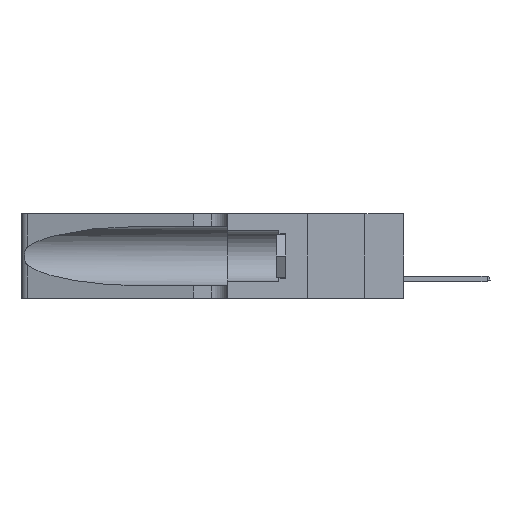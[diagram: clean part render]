
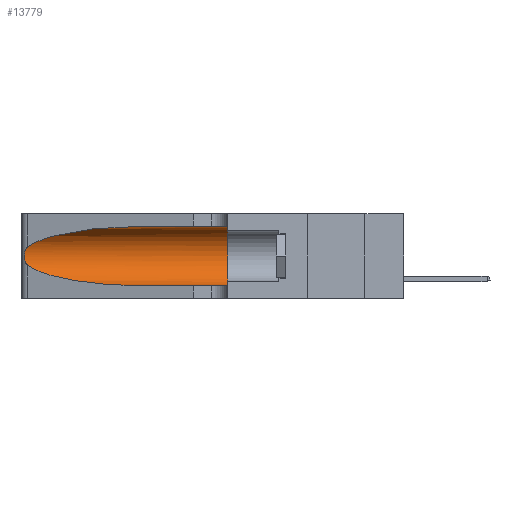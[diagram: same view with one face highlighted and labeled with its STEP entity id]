
A CAD part, left-side view. The second image highlights one B-rep face of the part: STEP entity #13779.
In plain terms, the highlighted cylindrical face has radius 3.308 mm (diameter 6.617 mm), a partial arc.
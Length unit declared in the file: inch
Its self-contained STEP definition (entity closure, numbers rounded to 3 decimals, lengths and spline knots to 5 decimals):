
#1563 = CIRCLE ( 'NONE', #30431, 0.13025 ) ;
#2128 = DIRECTION ( 'NONE',  ( 0., -1., 0. ) ) ;
#2639 = CARTESIAN_POINT ( 'NONE',  ( 0.1305, 0.72297, 0.05475 ) ) ;
#2937 = LINE ( 'NONE', #25227, #20079 ) ;
#3368 = CARTESIAN_POINT ( 'NONE',  ( 0.25487, 1.22718, 0.22369 ) ) ;
#3842 = VECTOR ( 'NONE', #2128, 39.37008 ) ;
#4030 = CARTESIAN_POINT ( 'NONE',  ( 0.1305, 1.61858, 0.185 ) ) ;
#4147 = DIRECTION ( 'NONE',  ( 0., 0., -1. ) ) ;
#4470 = VERTEX_POINT ( 'NONE', #21266 ) ;
#5541 = EDGE_CURVE ( 'NONE', #15825, #21465, #2937, .T. ) ;
#6198 = CARTESIAN_POINT ( 'NONE',  ( 0.26018, 1.23835, 0.19895 ) ) ;
#6557 = FACE_OUTER_BOUND ( 'NONE', #30679, .T. ) ;
#7634 = CARTESIAN_POINT ( 'NONE',  ( 0.1305, 0.72297, 0.31525 ) ) ;
#8065 = EDGE_CURVE ( 'NONE', #4470, #16647, #25391, .T. ) ;
#8548 = ORIENTED_EDGE ( 'NONE', *, *, #5541, .T. ) ;
#8876 = CARTESIAN_POINT ( 'NONE',  ( 0.26017, 1.23833, 0.17102 ) ) ;
#9345 = CARTESIAN_POINT ( 'NONE',  ( 0.1305, 0.35, 0.31525 ) ) ;
#9845 = DIRECTION ( 'NONE',  ( 0., 0., 1. ) ) ;
#10016 = CARTESIAN_POINT ( 'NONE',  ( 0.2373, 1.15595, 0.28018 ) ) ;
#11041 = CARTESIAN_POINT ( 'NONE',  ( 0.26075, 1.23896, 0.178 ) ) ;
#11052 = EDGE_CURVE ( 'NONE', #28292, #21465, #1563, .T. ) ;
#11179 = DIRECTION ( 'NONE',  ( 0., -1., 0. ) ) ;
#12004 =( BOUNDED_CURVE ( )  B_SPLINE_CURVE ( 3, ( #7634, #24281, #10016, #15506 ),
 .UNSPECIFIED., .F., .F. ) 
 B_SPLINE_CURVE_WITH_KNOTS ( ( 4, 4 ),
 ( 1.5708, 2.84003 ),
 .UNSPECIFIED. ) 
 CURVE ( )  GEOMETRIC_REPRESENTATION_ITEM ( )  RATIONAL_B_SPLINE_CURVE ( ( 1., 0.87, 0.87, 1. ) ) 
 REPRESENTATION_ITEM ( '' )  );
#12706 = CARTESIAN_POINT ( 'NONE',  ( 0.25555, 1.22994, 0.2215 ) ) ;
#12794 = ORIENTED_EDGE ( 'NONE', *, *, #8065, .T. ) ;
#13779 = ADVANCED_FACE ( 'NONE', ( #6557 ), #30365, .F. ) ;
#14035 = CARTESIAN_POINT ( 'NONE',  ( 0.25639, 1.23186, 0.15144 ) ) ;
#15506 = CARTESIAN_POINT ( 'NONE',  ( 0.25487, 1.22718, 0.22369 ) ) ;
#15825 = VERTEX_POINT ( 'NONE', #2639 ) ;
#16026 = CARTESIAN_POINT ( 'NONE',  ( 0.25487, 1.22718, 0.14631 ) ) ;
#16577 = ORIENTED_EDGE ( 'NONE', *, *, #24118, .T. ) ;
#16587 =( BOUNDED_CURVE ( )  B_SPLINE_CURVE ( 3, ( #16972, #24172, #19487, #16879 ),
 .UNSPECIFIED., .F., .T. ) 
 B_SPLINE_CURVE_WITH_KNOTS ( ( 4, 4 ),
 ( 3.44316, 4.71239 ),
 .UNSPECIFIED. ) 
 CURVE ( )  GEOMETRIC_REPRESENTATION_ITEM ( )  RATIONAL_B_SPLINE_CURVE ( ( 1., 0.87, 0.87, 1. ) ) 
 REPRESENTATION_ITEM ( '' )  );
#16647 = VERTEX_POINT ( 'NONE', #20194 ) ;
#16879 = CARTESIAN_POINT ( 'NONE',  ( 0.1305, 0.72297, 0.05475 ) ) ;
#16972 = CARTESIAN_POINT ( 'NONE',  ( 0.25487, 1.22718, 0.14631 ) ) ;
#17222 = EDGE_CURVE ( 'NONE', #27846, #4470, #12004, .T. ) ;
#17289 = EDGE_CURVE ( 'NONE', #27846, #28292, #20924, .T. ) ;
#17446 = CARTESIAN_POINT ( 'NONE',  ( 0.1305, 0.72297, 0.31525 ) ) ;
#19487 = CARTESIAN_POINT ( 'NONE',  ( 0.18966, 0.96281, 0.05475 ) ) ;
#19580 = CARTESIAN_POINT ( 'NONE',  ( 0.1305, 0.35, 0.05475 ) ) ;
#20002 = CARTESIAN_POINT ( 'NONE',  ( 0.25639, 1.23184, 0.21858 ) ) ;
#20079 = VECTOR ( 'NONE', #20534, 39.37008 ) ;
#20194 = CARTESIAN_POINT ( 'NONE',  ( 0.25487, 1.22718, 0.14631 ) ) ;
#20534 = DIRECTION ( 'NONE',  ( 0., -1., 0. ) ) ;
#20621 = ORIENTED_EDGE ( 'NONE', *, *, #17289, .F. ) ;
#20924 = LINE ( 'NONE', #30333, #3842 ) ;
#21003 = ORIENTED_EDGE ( 'NONE', *, *, #11052, .F. ) ;
#21218 = CARTESIAN_POINT ( 'NONE',  ( 0.1305, 0.35, 0.185 ) ) ;
#21233 = CARTESIAN_POINT ( 'NONE',  ( 0.25555, 1.22993, 0.14849 ) ) ;
#21266 = CARTESIAN_POINT ( 'NONE',  ( 0.25487, 1.22718, 0.22369 ) ) ;
#21465 = VERTEX_POINT ( 'NONE', #19580 ) ;
#22715 = CARTESIAN_POINT ( 'NONE',  ( 0.25856, 1.23593, 0.16098 ) ) ;
#23422 = DIRECTION ( 'NONE',  ( 0., 1., 0. ) ) ;
#24118 = EDGE_CURVE ( 'NONE', #16647, #15825, #16587, .T. ) ;
#24172 = CARTESIAN_POINT ( 'NONE',  ( 0.2373, 1.15595, 0.08982 ) ) ;
#24281 = CARTESIAN_POINT ( 'NONE',  ( 0.18966, 0.96281, 0.31525 ) ) ;
#24809 = CARTESIAN_POINT ( 'NONE',  ( 0.25854, 1.2359, 0.20912 ) ) ;
#25227 = CARTESIAN_POINT ( 'NONE',  ( 0.1305, 1.61858, 0.05475 ) ) ;
#25321 = CARTESIAN_POINT ( 'NONE',  ( 0.26075, 1.23896, 0.19203 ) ) ;
#25391 = B_SPLINE_CURVE_WITH_KNOTS ( 'NONE', 3,
 ( #3368, #12706, #20002, #29399, #24809, #6198, #25321, #11041, #8876, #22715, #27714, #14035, #21233, #16026 ),
 .UNSPECIFIED., .F., .F.,
 ( 4, 2, 2, 2, 2, 2, 4 ),
 ( 0., 0.00027, 0.00053, 0.00107, 0.0016, 0.00187, 0.00214 ),
 .UNSPECIFIED. ) ;
#25664 = AXIS2_PLACEMENT_3D ( 'NONE', #4030, #11179, #4147 ) ;
#27714 = CARTESIAN_POINT ( 'NONE',  ( 0.25789, 1.23486, 0.15765 ) ) ;
#27846 = VERTEX_POINT ( 'NONE', #17446 ) ;
#28292 = VERTEX_POINT ( 'NONE', #9345 ) ;
#29399 = CARTESIAN_POINT ( 'NONE',  ( 0.25787, 1.23484, 0.2124 ) ) ;
#30333 = CARTESIAN_POINT ( 'NONE',  ( 0.1305, 1.61858, 0.31525 ) ) ;
#30365 = CYLINDRICAL_SURFACE ( 'NONE', #25664, 0.13025 ) ;
#30431 = AXIS2_PLACEMENT_3D ( 'NONE', #21218, #23422, #9845 ) ;
#30619 = ORIENTED_EDGE ( 'NONE', *, *, #17222, .T. ) ;
#30679 = EDGE_LOOP ( 'NONE', ( #30619, #12794, #16577, #8548, #21003, #20621 ) ) ;
